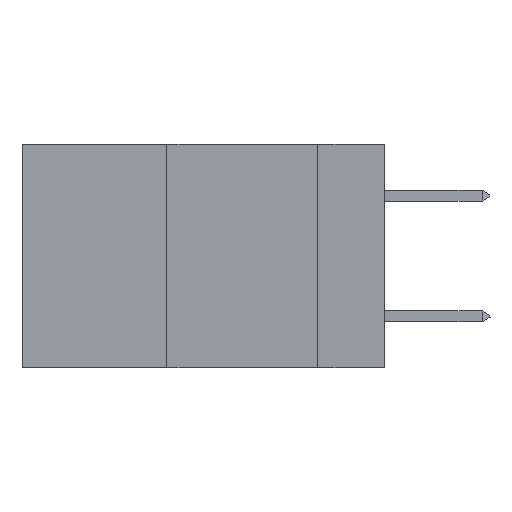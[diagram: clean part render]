
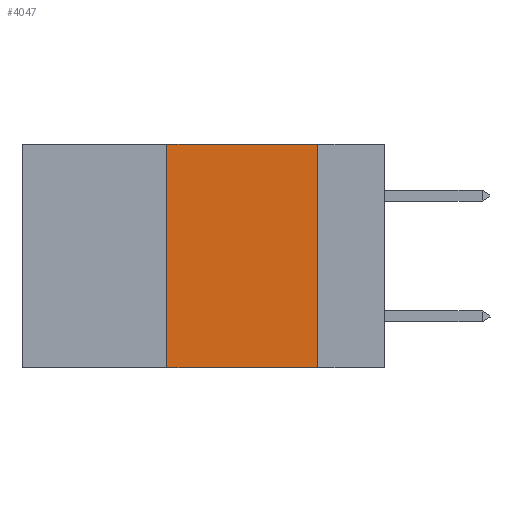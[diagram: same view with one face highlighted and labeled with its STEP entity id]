
A CAD part, left-side view. The second image highlights one B-rep face of the part: STEP entity #4047.
In plain terms, the highlighted planar face has unit normal (-1, 0, 0).
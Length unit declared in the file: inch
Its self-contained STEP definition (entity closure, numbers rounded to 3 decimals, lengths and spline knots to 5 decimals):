
#516 = VECTOR ( 'NONE', #1195, 39.37008 ) ;
#1195 = DIRECTION ( 'NONE',  ( 0., -1., 0. ) ) ;
#1867 = LINE ( 'NONE', #3949, #14883 ) ;
#2023 = VERTEX_POINT ( 'NONE', #15555 ) ;
#2616 = VERTEX_POINT ( 'NONE', #7627 ) ;
#3300 = ORIENTED_EDGE ( 'NONE', *, *, #6691, .T. ) ;
#3949 = CARTESIAN_POINT ( 'NONE',  ( 0., 0.6, -0.37 ) ) ;
#4047 = ADVANCED_FACE ( 'NONE', ( #4336 ), #14132, .F. ) ;
#4312 = CARTESIAN_POINT ( 'NONE',  ( 0., 0.36, 0. ) ) ;
#4336 = FACE_OUTER_BOUND ( 'NONE', #10945, .T. ) ;
#4369 = EDGE_CURVE ( 'NONE', #8920, #2023, #6343, .T. ) ;
#5430 = CARTESIAN_POINT ( 'NONE',  ( 0., 0.11, 0. ) ) ;
#5711 = ORIENTED_EDGE ( 'NONE', *, *, #9136, .F. ) ;
#5787 = ORIENTED_EDGE ( 'NONE', *, *, #4369, .F. ) ;
#6343 = LINE ( 'NONE', #4312, #9384 ) ;
#6350 = DIRECTION ( 'NONE',  ( 1., 0., 0. ) ) ;
#6691 = EDGE_CURVE ( 'NONE', #8920, #15398, #1867, .T. ) ;
#6734 = DIRECTION ( 'NONE',  ( 0., 0., -1. ) ) ;
#6910 = DIRECTION ( 'NONE',  ( 0., 0., 1. ) ) ;
#7618 = CARTESIAN_POINT ( 'NONE',  ( 0., 0.6, 0. ) ) ;
#7627 = CARTESIAN_POINT ( 'NONE',  ( 0., 0.11, 0. ) ) ;
#8426 = ORIENTED_EDGE ( 'NONE', *, *, #11932, .F. ) ;
#8517 = VECTOR ( 'NONE', #6734, 39.37008 ) ;
#8920 = VERTEX_POINT ( 'NONE', #10217 ) ;
#8927 = LINE ( 'NONE', #5430, #8517 ) ;
#9136 = EDGE_CURVE ( 'NONE', #2616, #15398, #8927, .T. ) ;
#9384 = VECTOR ( 'NONE', #6910, 39.37008 ) ;
#10217 = CARTESIAN_POINT ( 'NONE',  ( 0., 0.36, -0.37 ) ) ;
#10866 = LINE ( 'NONE', #7618, #516 ) ;
#10945 = EDGE_LOOP ( 'NONE', ( #5711, #8426, #5787, #3300 ) ) ;
#11511 = CARTESIAN_POINT ( 'NONE',  ( 0., 0.6, 0. ) ) ;
#11932 = EDGE_CURVE ( 'NONE', #2023, #2616, #10866, .T. ) ;
#14132 = PLANE ( 'NONE',  #15337 ) ;
#14331 = DIRECTION ( 'NONE',  ( 0., -1., 0. ) ) ;
#14512 = CARTESIAN_POINT ( 'NONE',  ( 0., 0.11, -0.37 ) ) ;
#14883 = VECTOR ( 'NONE', #14331, 39.37008 ) ;
#15337 = AXIS2_PLACEMENT_3D ( 'NONE', #11511, #6350, #15472 ) ;
#15398 = VERTEX_POINT ( 'NONE', #14512 ) ;
#15472 = DIRECTION ( 'NONE',  ( 0., 0., -1. ) ) ;
#15555 = CARTESIAN_POINT ( 'NONE',  ( 0., 0.36, 0. ) ) ;
